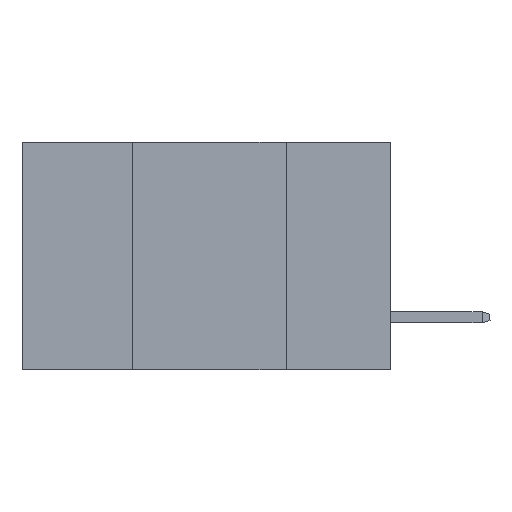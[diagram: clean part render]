
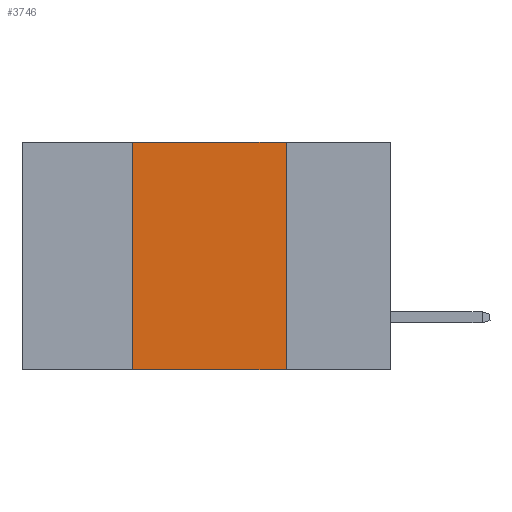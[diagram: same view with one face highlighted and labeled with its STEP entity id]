
A CAD part, left-side view. The second image highlights one B-rep face of the part: STEP entity #3746.
In plain terms, the highlighted planar face has unit normal (-1, 0, 0).
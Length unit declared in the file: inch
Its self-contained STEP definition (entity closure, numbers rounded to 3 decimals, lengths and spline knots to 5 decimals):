
#286 = CARTESIAN_POINT ( 'NONE',  ( 0., 0.42, 0. ) ) ;
#1068 = DIRECTION ( 'NONE',  ( 0., 0., 1. ) ) ;
#1096 = VERTEX_POINT ( 'NONE', #5857 ) ;
#1595 = DIRECTION ( 'NONE',  ( 1., 0., 0. ) ) ;
#1634 = CARTESIAN_POINT ( 'NONE',  ( 0., 0.6, 0. ) ) ;
#1752 = EDGE_CURVE ( 'NONE', #4075, #2074, #5877, .T. ) ;
#2056 = VECTOR ( 'NONE', #4908, 39.37008 ) ;
#2074 = VERTEX_POINT ( 'NONE', #9732 ) ;
#2302 = ORIENTED_EDGE ( 'NONE', *, *, #2981, .T. ) ;
#2651 = LINE ( 'NONE', #4720, #5221 ) ;
#2981 = EDGE_CURVE ( 'NONE', #4075, #1096, #2651, .T. ) ;
#3177 = CARTESIAN_POINT ( 'NONE',  ( 0., 0.17, 0. ) ) ;
#3497 = CARTESIAN_POINT ( 'NONE',  ( 0., 0.6, 0. ) ) ;
#3680 = VERTEX_POINT ( 'NONE', #3177 ) ;
#3746 = ADVANCED_FACE ( 'NONE', ( #5455 ), #6308, .F. ) ;
#3896 = DIRECTION ( 'NONE',  ( 0., -1., 0. ) ) ;
#4000 = EDGE_LOOP ( 'NONE', ( #6714, #6876, #7605, #2302 ) ) ;
#4075 = VERTEX_POINT ( 'NONE', #5229 ) ;
#4512 = VECTOR ( 'NONE', #4552, 39.37008 ) ;
#4552 = DIRECTION ( 'NONE',  ( 0., 0., -1. ) ) ;
#4720 = CARTESIAN_POINT ( 'NONE',  ( 0., 0.6, -0.37 ) ) ;
#4908 = DIRECTION ( 'NONE',  ( 0., -1., 0. ) ) ;
#5033 = AXIS2_PLACEMENT_3D ( 'NONE', #1634, #1595, #7107 ) ;
#5221 = VECTOR ( 'NONE', #3896, 39.37008 ) ;
#5229 = CARTESIAN_POINT ( 'NONE',  ( 0., 0.42, -0.37 ) ) ;
#5235 = LINE ( 'NONE', #3497, #2056 ) ;
#5455 = FACE_OUTER_BOUND ( 'NONE', #4000, .T. ) ;
#5857 = CARTESIAN_POINT ( 'NONE',  ( 0., 0.17, -0.37 ) ) ;
#5877 = LINE ( 'NONE', #286, #8432 ) ;
#6308 = PLANE ( 'NONE',  #5033 ) ;
#6714 = ORIENTED_EDGE ( 'NONE', *, *, #8122, .F. ) ;
#6724 = CARTESIAN_POINT ( 'NONE',  ( 0., 0.17, 0. ) ) ;
#6876 = ORIENTED_EDGE ( 'NONE', *, *, #8704, .F. ) ;
#7107 = DIRECTION ( 'NONE',  ( 0., 0., -1. ) ) ;
#7605 = ORIENTED_EDGE ( 'NONE', *, *, #1752, .F. ) ;
#8122 = EDGE_CURVE ( 'NONE', #3680, #1096, #9053, .T. ) ;
#8432 = VECTOR ( 'NONE', #1068, 39.37008 ) ;
#8704 = EDGE_CURVE ( 'NONE', #2074, #3680, #5235, .T. ) ;
#9053 = LINE ( 'NONE', #6724, #4512 ) ;
#9732 = CARTESIAN_POINT ( 'NONE',  ( 0., 0.42, 0. ) ) ;
